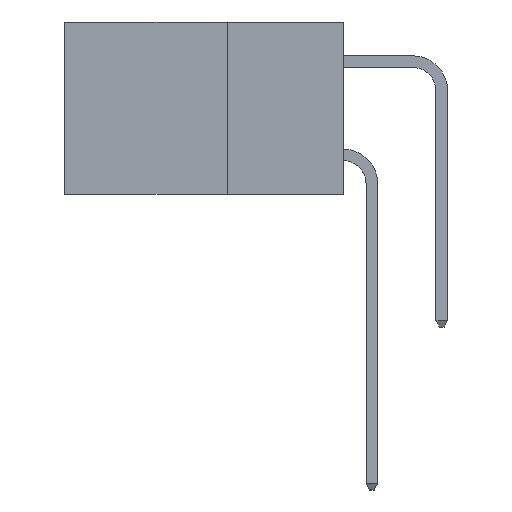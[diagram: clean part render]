
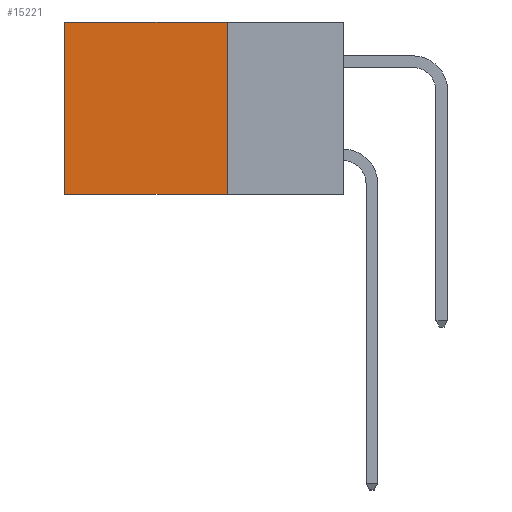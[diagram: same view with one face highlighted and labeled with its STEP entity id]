
A CAD part, left-side view. The second image highlights one B-rep face of the part: STEP entity #15221.
In plain terms, the highlighted planar face has unit normal (-1, 0, 0).
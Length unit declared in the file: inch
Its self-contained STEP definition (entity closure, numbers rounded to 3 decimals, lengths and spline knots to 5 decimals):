
#1222 = LINE ( 'NONE', #16178, #11456 ) ;
#1326 = DIRECTION ( 'NONE',  ( 0., 0., -1. ) ) ;
#1669 = DIRECTION ( 'NONE',  ( 0., 1., 0. ) ) ;
#1696 = CARTESIAN_POINT ( 'NONE',  ( 0.2615, 0.25, 0. ) ) ;
#1772 = DIRECTION ( 'NONE',  ( 0., 1., 0. ) ) ;
#1774 = VECTOR ( 'NONE', #2880, 39.37008 ) ;
#2550 = CARTESIAN_POINT ( 'NONE',  ( 0.2615, 0.6, -0.37 ) ) ;
#2880 = DIRECTION ( 'NONE',  ( 0., 0., -1. ) ) ;
#3020 = VERTEX_POINT ( 'NONE', #3848 ) ;
#3683 = EDGE_CURVE ( 'NONE', #15082, #3020, #16734, .T. ) ;
#3848 = CARTESIAN_POINT ( 'NONE',  ( 0.2615, 0.6, 0. ) ) ;
#5363 = PLANE ( 'NONE',  #7777 ) ;
#5741 = EDGE_CURVE ( 'NONE', #3020, #11726, #8916, .T. ) ;
#6477 = VECTOR ( 'NONE', #1772, 39.37008 ) ;
#7777 = AXIS2_PLACEMENT_3D ( 'NONE', #16982, #9370, #1326 ) ;
#7866 = ORIENTED_EDGE ( 'NONE', *, *, #3683, .T. ) ;
#8916 = LINE ( 'NONE', #2550, #1774 ) ;
#9229 = VECTOR ( 'NONE', #15123, 39.37008 ) ;
#9370 = DIRECTION ( 'NONE',  ( 1., 0., 0. ) ) ;
#9721 = CARTESIAN_POINT ( 'NONE',  ( 0.2615, 0.25, -0.37 ) ) ;
#11456 = VECTOR ( 'NONE', #1669, 39.37008 ) ;
#11591 = ORIENTED_EDGE ( 'NONE', *, *, #5741, .T. ) ;
#11726 = VERTEX_POINT ( 'NONE', #15443 ) ;
#12075 = VERTEX_POINT ( 'NONE', #9721 ) ;
#12184 = ORIENTED_EDGE ( 'NONE', *, *, #15705, .F. ) ;
#12220 = EDGE_CURVE ( 'NONE', #15082, #12075, #12729, .T. ) ;
#12729 = LINE ( 'NONE', #13848, #9229 ) ;
#13185 = ORIENTED_EDGE ( 'NONE', *, *, #12220, .F. ) ;
#13848 = CARTESIAN_POINT ( 'NONE',  ( 0.2615, 0.25, -0.37 ) ) ;
#15082 = VERTEX_POINT ( 'NONE', #15334 ) ;
#15123 = DIRECTION ( 'NONE',  ( 0., 0., -1. ) ) ;
#15221 = ADVANCED_FACE ( 'NONE', ( #16555 ), #5363, .F. ) ;
#15334 = CARTESIAN_POINT ( 'NONE',  ( 0.2615, 0.25, 0. ) ) ;
#15424 = EDGE_LOOP ( 'NONE', ( #11591, #12184, #13185, #7866 ) ) ;
#15443 = CARTESIAN_POINT ( 'NONE',  ( 0.2615, 0.6, -0.37 ) ) ;
#15705 = EDGE_CURVE ( 'NONE', #12075, #11726, #1222, .T. ) ;
#16178 = CARTESIAN_POINT ( 'NONE',  ( 0.2615, 0.25, -0.37 ) ) ;
#16555 = FACE_OUTER_BOUND ( 'NONE', #15424, .T. ) ;
#16734 = LINE ( 'NONE', #1696, #6477 ) ;
#16982 = CARTESIAN_POINT ( 'NONE',  ( 0.2615, 0.25, -0.37 ) ) ;
